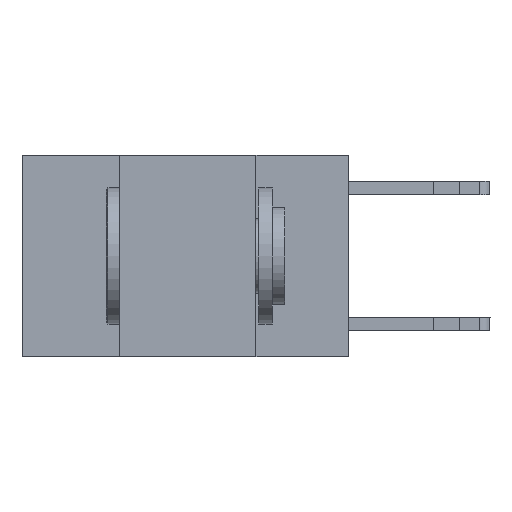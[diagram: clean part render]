
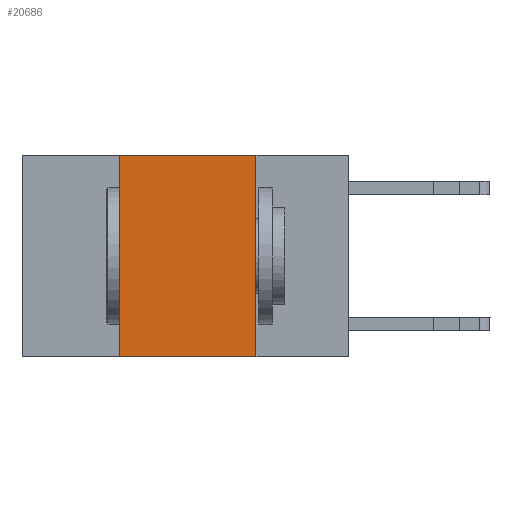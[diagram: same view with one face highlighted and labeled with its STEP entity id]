
A CAD part, left-side view. The second image highlights one B-rep face of the part: STEP entity #20686.
In plain terms, the highlighted planar face has unit normal (-1, 0, 0).
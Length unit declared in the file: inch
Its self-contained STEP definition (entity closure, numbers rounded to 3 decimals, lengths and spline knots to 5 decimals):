
#753 = ORIENTED_EDGE ( 'NONE', *, *, #2166, .F. ) ;
#830 = CARTESIAN_POINT ( 'NONE',  ( 0., 0.17, -0.37 ) ) ;
#1711 = VECTOR ( 'NONE', #18915, 39.37008 ) ;
#2166 = EDGE_CURVE ( 'NONE', #18946, #16739, #5899, .T. ) ;
#2566 = AXIS2_PLACEMENT_3D ( 'NONE', #13037, #23971, #19859 ) ;
#3699 = VERTEX_POINT ( 'NONE', #830 ) ;
#4579 = EDGE_LOOP ( 'NONE', ( #21492, #753, #18290, #12826 ) ) ;
#4684 = FACE_OUTER_BOUND ( 'NONE', #4579, .T. ) ;
#5428 = EDGE_CURVE ( 'NONE', #16739, #3699, #14818, .T. ) ;
#5497 = DIRECTION ( 'NONE',  ( 0., -1., 0. ) ) ;
#5899 = LINE ( 'NONE', #9887, #9793 ) ;
#7431 = EDGE_CURVE ( 'NONE', #16436, #3699, #17726, .T. ) ;
#9793 = VECTOR ( 'NONE', #5497, 39.37008 ) ;
#9887 = CARTESIAN_POINT ( 'NONE',  ( 0., 0.6, 0. ) ) ;
#11745 = VECTOR ( 'NONE', #19506, 39.37008 ) ;
#11901 = CARTESIAN_POINT ( 'NONE',  ( 0., 0.17, 0. ) ) ;
#12102 = CARTESIAN_POINT ( 'NONE',  ( 0., 0.42, -0.37 ) ) ;
#12215 = CARTESIAN_POINT ( 'NONE',  ( 0., 0.17, 0. ) ) ;
#12826 = ORIENTED_EDGE ( 'NONE', *, *, #7431, .T. ) ;
#13037 = CARTESIAN_POINT ( 'NONE',  ( 0., 0.6, 0. ) ) ;
#13435 = PLANE ( 'NONE',  #2566 ) ;
#13610 = CARTESIAN_POINT ( 'NONE',  ( 0., 0.6, -0.37 ) ) ;
#13878 = VECTOR ( 'NONE', #14440, 39.37008 ) ;
#14440 = DIRECTION ( 'NONE',  ( 0., 0., 1. ) ) ;
#14818 = LINE ( 'NONE', #12215, #1711 ) ;
#16436 = VERTEX_POINT ( 'NONE', #12102 ) ;
#16739 = VERTEX_POINT ( 'NONE', #11901 ) ;
#17726 = LINE ( 'NONE', #13610, #11745 ) ;
#18290 = ORIENTED_EDGE ( 'NONE', *, *, #19139, .F. ) ;
#18915 = DIRECTION ( 'NONE',  ( 0., 0., -1. ) ) ;
#18946 = VERTEX_POINT ( 'NONE', #19921 ) ;
#19139 = EDGE_CURVE ( 'NONE', #16436, #18946, #26617, .T. ) ;
#19506 = DIRECTION ( 'NONE',  ( 0., -1., 0. ) ) ;
#19859 = DIRECTION ( 'NONE',  ( 0., 0., -1. ) ) ;
#19921 = CARTESIAN_POINT ( 'NONE',  ( 0., 0.42, 0. ) ) ;
#20686 = ADVANCED_FACE ( 'NONE', ( #4684 ), #13435, .F. ) ;
#21006 = CARTESIAN_POINT ( 'NONE',  ( 0., 0.42, 0. ) ) ;
#21492 = ORIENTED_EDGE ( 'NONE', *, *, #5428, .F. ) ;
#23971 = DIRECTION ( 'NONE',  ( 1., 0., 0. ) ) ;
#26617 = LINE ( 'NONE', #21006, #13878 ) ;
